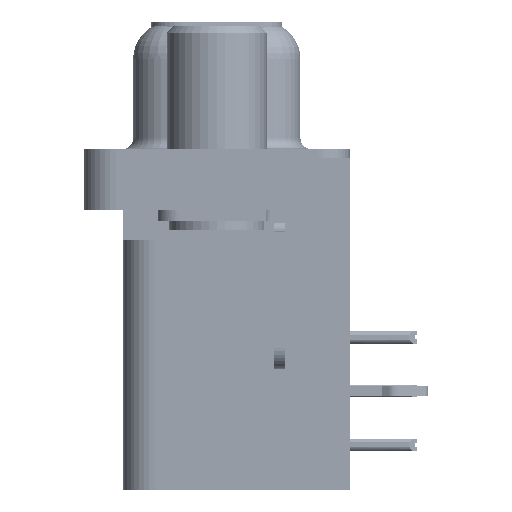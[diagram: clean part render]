
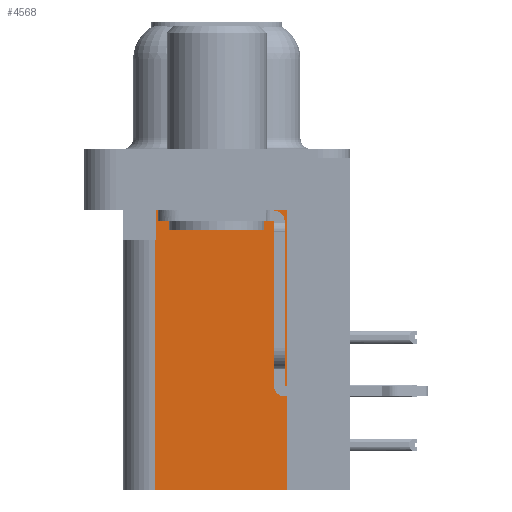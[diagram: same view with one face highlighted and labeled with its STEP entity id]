
A CAD part, left-side view. The second image highlights one B-rep face of the part: STEP entity #4568.
In plain terms, the highlighted planar face has unit normal (-1, 0, 0).
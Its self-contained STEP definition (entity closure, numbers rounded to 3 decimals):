
#379 = ORIENTED_EDGE ( 'NONE', *, *, #15181, .T. ) ;
#1302 = ORIENTED_EDGE ( 'NONE', *, *, #21625, .T. ) ;
#4568 = ADVANCED_FACE ( 'NONE', ( #11739 ), #37888, .F. ) ;
#4747 = EDGE_CURVE ( 'NONE', #32811, #23871, #10473, .T. ) ;
#4811 = DIRECTION ( 'NONE',  ( 0., 1., 0. ) ) ;
#10425 = VECTOR ( 'NONE', #40363, 1000. ) ;
#10473 = LINE ( 'NONE', #41135, #10425 ) ;
#11611 = VERTEX_POINT ( 'NONE', #19560 ) ;
#11645 = LINE ( 'NONE', #11968, #11806 ) ;
#11678 = CARTESIAN_POINT ( 'NONE',  ( 3.7, -3.295, -15.7 ) ) ;
#11739 = FACE_OUTER_BOUND ( 'NONE', #30364, .T. ) ;
#11806 = VECTOR ( 'NONE', #4811, 1000. ) ;
#11968 = CARTESIAN_POINT ( 'NONE',  ( 3.7, -3.295, -2.5 ) ) ;
#12530 = AXIS2_PLACEMENT_3D ( 'NONE', #36102, #34447, #34306 ) ;
#14898 = CARTESIAN_POINT ( 'NONE',  ( 3.7, -3.295, -2.5 ) ) ;
#15181 = EDGE_CURVE ( 'NONE', #21408, #11611, #11645, .T. ) ;
#16882 = ORIENTED_EDGE ( 'NONE', *, *, #4747, .T. ) ;
#17052 = VERTEX_POINT ( 'NONE', #38310 ) ;
#18399 = VECTOR ( 'NONE', #23012, 1000. ) ;
#19098 = LINE ( 'NONE', #40574, #18399 ) ;
#19560 = CARTESIAN_POINT ( 'NONE',  ( 3.7, 2.895, -2.5 ) ) ;
#21408 = VERTEX_POINT ( 'NONE', #14898 ) ;
#21625 = EDGE_CURVE ( 'NONE', #11611, #32811, #45389, .T. ) ;
#23012 = DIRECTION ( 'NONE',  ( 0., 1., 0. ) ) ;
#23094 = ORIENTED_EDGE ( 'NONE', *, *, #24794, .F. ) ;
#23871 = VERTEX_POINT ( 'NONE', #35095 ) ;
#24794 = EDGE_CURVE ( 'NONE', #17052, #23871, #27471, .T. ) ;
#27314 = VECTOR ( 'NONE', #41282, 1000. ) ;
#27471 = LINE ( 'NONE', #37729, #27314 ) ;
#29178 = VECTOR ( 'NONE', #32902, 1000. ) ;
#29325 = LINE ( 'NONE', #11678, #29178 ) ;
#30364 = EDGE_LOOP ( 'NONE', ( #379, #1302, #16882, #23094, #38077, #40497 ) ) ;
#32811 = VERTEX_POINT ( 'NONE', #34158 ) ;
#32902 = DIRECTION ( 'NONE',  ( 0., 0., 1. ) ) ;
#33998 = CARTESIAN_POINT ( 'NONE',  ( 3.7, 2.895, -3.9 ) ) ;
#34158 = CARTESIAN_POINT ( 'NONE',  ( 3.7, 2.895, -3.9 ) ) ;
#34306 = DIRECTION ( 'NONE',  ( 0., 1., 0. ) ) ;
#34447 = DIRECTION ( 'NONE',  ( 1., 0., 0. ) ) ;
#35095 = CARTESIAN_POINT ( 'NONE',  ( 3.7, 2.925, -3.9 ) ) ;
#36001 = EDGE_CURVE ( 'NONE', #43345, #21408, #29325, .T. ) ;
#36102 = CARTESIAN_POINT ( 'NONE',  ( 3.7, -3.295, -15.7 ) ) ;
#37442 = DIRECTION ( 'NONE',  ( 0., 0., -1. ) ) ;
#37729 = CARTESIAN_POINT ( 'NONE',  ( 3.7, 2.925, -15.7 ) ) ;
#37888 = PLANE ( 'NONE',  #12530 ) ;
#38077 = ORIENTED_EDGE ( 'NONE', *, *, #43049, .F. ) ;
#38310 = CARTESIAN_POINT ( 'NONE',  ( 3.7, 2.925, -15.7 ) ) ;
#39060 = CARTESIAN_POINT ( 'NONE',  ( 3.7, -3.295, -15.7 ) ) ;
#40363 = DIRECTION ( 'NONE',  ( 0., 1., 0. ) ) ;
#40497 = ORIENTED_EDGE ( 'NONE', *, *, #36001, .T. ) ;
#40574 = CARTESIAN_POINT ( 'NONE',  ( 3.7, -3.295, -15.7 ) ) ;
#41135 = CARTESIAN_POINT ( 'NONE',  ( 3.7, 0., -3.9 ) ) ;
#41282 = DIRECTION ( 'NONE',  ( 0., 0., 1. ) ) ;
#43049 = EDGE_CURVE ( 'NONE', #43345, #17052, #19098, .T. ) ;
#43345 = VERTEX_POINT ( 'NONE', #39060 ) ;
#45292 = VECTOR ( 'NONE', #37442, 1000. ) ;
#45389 = LINE ( 'NONE', #33998, #45292 ) ;
